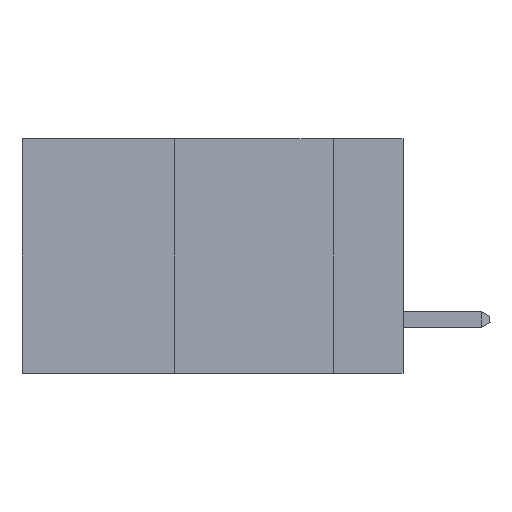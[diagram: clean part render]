
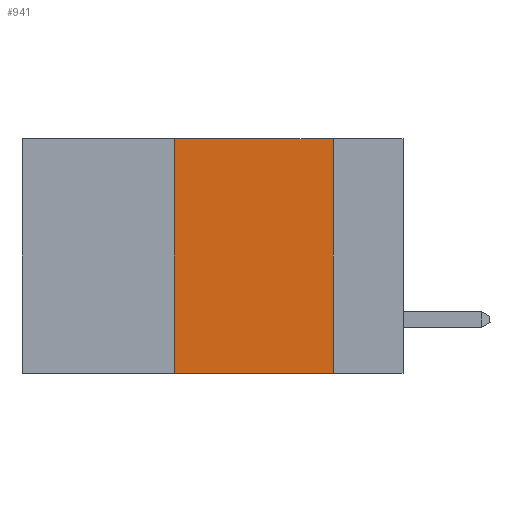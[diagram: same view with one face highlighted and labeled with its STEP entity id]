
A CAD part, left-side view. The second image highlights one B-rep face of the part: STEP entity #941.
In plain terms, the highlighted planar face has unit normal (-1, 0, 0).
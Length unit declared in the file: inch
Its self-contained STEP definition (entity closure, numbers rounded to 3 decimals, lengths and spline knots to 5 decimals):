
#37 = LINE ( 'NONE', #21116, #1976 ) ;
#297 = ORIENTED_EDGE ( 'NONE', *, *, #26759, .T. ) ;
#941 = ADVANCED_FACE ( 'NONE', ( #3516 ), #14197, .F. ) ;
#958 = CARTESIAN_POINT ( 'NONE',  ( 0., 0.11, 0. ) ) ;
#971 = LINE ( 'NONE', #14958, #5824 ) ;
#1317 = VECTOR ( 'NONE', #8825, 39.37008 ) ;
#1697 = CARTESIAN_POINT ( 'NONE',  ( 0., 0.11, -0.37 ) ) ;
#1976 = VECTOR ( 'NONE', #8974, 39.37008 ) ;
#3516 = FACE_OUTER_BOUND ( 'NONE', #12944, .T. ) ;
#4327 = DIRECTION ( 'NONE',  ( 0., -1., 0. ) ) ;
#4331 = VERTEX_POINT ( 'NONE', #958 ) ;
#5824 = VECTOR ( 'NONE', #4327, 39.37008 ) ;
#5850 = CARTESIAN_POINT ( 'NONE',  ( 0., 0.6, 0. ) ) ;
#6015 = DIRECTION ( 'NONE',  ( 1., 0., 0. ) ) ;
#7114 = EDGE_CURVE ( 'NONE', #15873, #4331, #15197, .T. ) ;
#7324 = ORIENTED_EDGE ( 'NONE', *, *, #7114, .F. ) ;
#7689 = VECTOR ( 'NONE', #23965, 39.37008 ) ;
#8106 = DIRECTION ( 'NONE',  ( 0., 0., -1. ) ) ;
#8825 = DIRECTION ( 'NONE',  ( 0., -1., 0. ) ) ;
#8974 = DIRECTION ( 'NONE',  ( 0., 0., -1. ) ) ;
#11288 = CARTESIAN_POINT ( 'NONE',  ( 0., 0.36, 0. ) ) ;
#12241 = ORIENTED_EDGE ( 'NONE', *, *, #16840, .F. ) ;
#12902 = CARTESIAN_POINT ( 'NONE',  ( 0., 0.36, -0.37 ) ) ;
#12944 = EDGE_LOOP ( 'NONE', ( #21325, #7324, #12241, #297 ) ) ;
#13196 = CARTESIAN_POINT ( 'NONE',  ( 0., 0.6, 0. ) ) ;
#13224 = LINE ( 'NONE', #11288, #7689 ) ;
#14197 = PLANE ( 'NONE',  #17683 ) ;
#14958 = CARTESIAN_POINT ( 'NONE',  ( 0., 0.6, -0.37 ) ) ;
#15197 = LINE ( 'NONE', #13196, #1317 ) ;
#15873 = VERTEX_POINT ( 'NONE', #21223 ) ;
#16840 = EDGE_CURVE ( 'NONE', #22027, #15873, #13224, .T. ) ;
#17683 = AXIS2_PLACEMENT_3D ( 'NONE', #5850, #6015, #8106 ) ;
#21116 = CARTESIAN_POINT ( 'NONE',  ( 0., 0.11, 0. ) ) ;
#21223 = CARTESIAN_POINT ( 'NONE',  ( 0., 0.36, 0. ) ) ;
#21325 = ORIENTED_EDGE ( 'NONE', *, *, #21964, .F. ) ;
#21964 = EDGE_CURVE ( 'NONE', #4331, #23550, #37, .T. ) ;
#22027 = VERTEX_POINT ( 'NONE', #12902 ) ;
#23550 = VERTEX_POINT ( 'NONE', #1697 ) ;
#23965 = DIRECTION ( 'NONE',  ( 0., 0., 1. ) ) ;
#26759 = EDGE_CURVE ( 'NONE', #22027, #23550, #971, .T. ) ;
